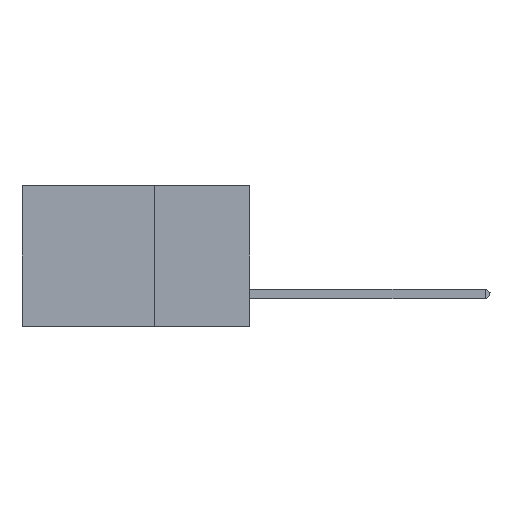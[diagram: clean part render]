
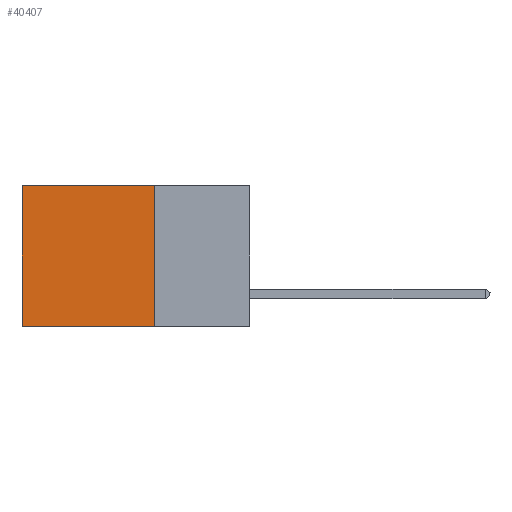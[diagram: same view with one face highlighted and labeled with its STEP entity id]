
A CAD part, left-side view. The second image highlights one B-rep face of the part: STEP entity #40407.
In plain terms, the highlighted planar face has unit normal (-1, 0, 0).
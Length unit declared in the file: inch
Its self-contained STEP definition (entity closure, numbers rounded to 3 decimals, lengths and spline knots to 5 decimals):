
#2979 = ORIENTED_EDGE ( 'NONE', *, *, #36315, .T. ) ;
#3577 = CARTESIAN_POINT ( 'NONE',  ( 0.2875, 0.25, -0.37 ) ) ;
#4446 = VERTEX_POINT ( 'NONE', #12776 ) ;
#5311 = CARTESIAN_POINT ( 'NONE',  ( 0.2875, 0.25, 0. ) ) ;
#5492 = LINE ( 'NONE', #5311, #7593 ) ;
#6931 = EDGE_CURVE ( 'NONE', #24323, #4446, #29032, .T. ) ;
#7216 = CARTESIAN_POINT ( 'NONE',  ( 0.2875, 0.25, 0. ) ) ;
#7593 = VECTOR ( 'NONE', #18061, 39.37008 ) ;
#11998 = VERTEX_POINT ( 'NONE', #30859 ) ;
#12776 = CARTESIAN_POINT ( 'NONE',  ( 0.2875, 0.6, -0.37 ) ) ;
#14306 = DIRECTION ( 'NONE',  ( 0., 0., -1. ) ) ;
#14867 = VECTOR ( 'NONE', #33099, 39.37008 ) ;
#15912 = PLANE ( 'NONE',  #39571 ) ;
#17107 = ORIENTED_EDGE ( 'NONE', *, *, #6931, .F. ) ;
#18061 = DIRECTION ( 'NONE',  ( 0., 1., 0. ) ) ;
#21396 = DIRECTION ( 'NONE',  ( 0., 0., -1. ) ) ;
#21786 = FACE_OUTER_BOUND ( 'NONE', #40678, .T. ) ;
#24323 = VERTEX_POINT ( 'NONE', #3577 ) ;
#24644 = VECTOR ( 'NONE', #14306, 39.37008 ) ;
#27414 = CARTESIAN_POINT ( 'NONE',  ( 0.2875, 0.25, 0. ) ) ;
#27743 = EDGE_CURVE ( 'NONE', #11998, #4446, #37212, .T. ) ;
#29032 = LINE ( 'NONE', #33230, #14867 ) ;
#30859 = CARTESIAN_POINT ( 'NONE',  ( 0.2875, 0.6, 0. ) ) ;
#32601 = ORIENTED_EDGE ( 'NONE', *, *, #43059, .F. ) ;
#33099 = DIRECTION ( 'NONE',  ( 0., 1., 0. ) ) ;
#33230 = CARTESIAN_POINT ( 'NONE',  ( 0.2875, 0.25, -0.37 ) ) ;
#34042 = LINE ( 'NONE', #27414, #24644 ) ;
#34047 = ORIENTED_EDGE ( 'NONE', *, *, #27743, .T. ) ;
#35629 = VECTOR ( 'NONE', #21396, 39.37008 ) ;
#36237 = DIRECTION ( 'NONE',  ( 1., 0., 0. ) ) ;
#36315 = EDGE_CURVE ( 'NONE', #39447, #11998, #5492, .T. ) ;
#36944 = DIRECTION ( 'NONE',  ( 0., 0., -1. ) ) ;
#37212 = LINE ( 'NONE', #38484, #35629 ) ;
#38484 = CARTESIAN_POINT ( 'NONE',  ( 0.2875, 0.6, 0. ) ) ;
#39447 = VERTEX_POINT ( 'NONE', #7216 ) ;
#39571 = AXIS2_PLACEMENT_3D ( 'NONE', #42792, #36237, #36944 ) ;
#40407 = ADVANCED_FACE ( 'NONE', ( #21786 ), #15912, .F. ) ;
#40678 = EDGE_LOOP ( 'NONE', ( #34047, #17107, #32601, #2979 ) ) ;
#42792 = CARTESIAN_POINT ( 'NONE',  ( 0.2875, 0.25, 0. ) ) ;
#43059 = EDGE_CURVE ( 'NONE', #39447, #24323, #34042, .T. ) ;
